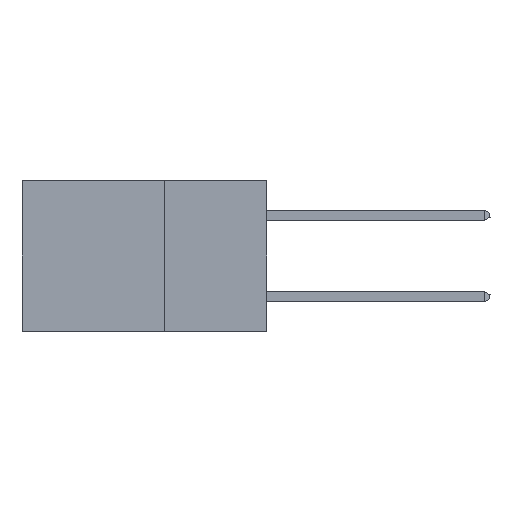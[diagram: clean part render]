
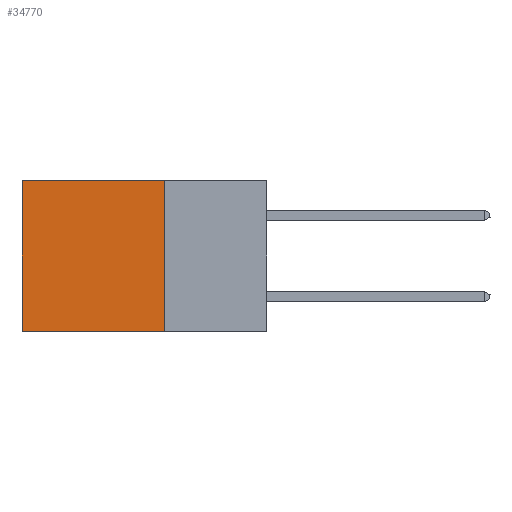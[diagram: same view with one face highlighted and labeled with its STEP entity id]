
A CAD part, left-side view. The second image highlights one B-rep face of the part: STEP entity #34770.
In plain terms, the highlighted planar face has unit normal (-1, 0, 0).
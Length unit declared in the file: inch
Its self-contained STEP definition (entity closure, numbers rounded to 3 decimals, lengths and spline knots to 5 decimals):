
#224 = LINE ( 'NONE', #38371, #41093 ) ;
#1330 = VECTOR ( 'NONE', #21002, 39.37008 ) ;
#1623 = DIRECTION ( 'NONE',  ( 0., 0., -1. ) ) ;
#4645 = CARTESIAN_POINT ( 'NONE',  ( 0.2875, 0.6, 0. ) ) ;
#5847 = CARTESIAN_POINT ( 'NONE',  ( 0.2875, 0.6, -0.37 ) ) ;
#6607 = LINE ( 'NONE', #7288, #1330 ) ;
#7288 = CARTESIAN_POINT ( 'NONE',  ( 0.2875, 0.6, 0. ) ) ;
#8214 = EDGE_CURVE ( 'NONE', #26000, #24510, #19349, .T. ) ;
#8493 = CARTESIAN_POINT ( 'NONE',  ( 0.2875, 0.25, 0. ) ) ;
#8495 = CARTESIAN_POINT ( 'NONE',  ( 0.2875, 0.25, 0. ) ) ;
#9388 = ORIENTED_EDGE ( 'NONE', *, *, #12309, .T. ) ;
#9783 = VERTEX_POINT ( 'NONE', #44958 ) ;
#10341 = EDGE_CURVE ( 'NONE', #9783, #12881, #25858, .T. ) ;
#10484 = CARTESIAN_POINT ( 'NONE',  ( 0.2875, 0.25, -0.37 ) ) ;
#12309 = EDGE_CURVE ( 'NONE', #12881, #24510, #6607, .T. ) ;
#12881 = VERTEX_POINT ( 'NONE', #4645 ) ;
#15265 = AXIS2_PLACEMENT_3D ( 'NONE', #8495, #32923, #1623 ) ;
#16148 = CARTESIAN_POINT ( 'NONE',  ( 0.2875, 0.25, -0.37 ) ) ;
#16545 = ORIENTED_EDGE ( 'NONE', *, *, #19852, .F. ) ;
#18821 = ORIENTED_EDGE ( 'NONE', *, *, #8214, .F. ) ;
#19349 = LINE ( 'NONE', #16148, #43800 ) ;
#19852 = EDGE_CURVE ( 'NONE', #9783, #26000, #224, .T. ) ;
#21002 = DIRECTION ( 'NONE',  ( 0., 0., -1. ) ) ;
#22776 = DIRECTION ( 'NONE',  ( 0., 1., 0. ) ) ;
#24510 = VERTEX_POINT ( 'NONE', #5847 ) ;
#25858 = LINE ( 'NONE', #8493, #29210 ) ;
#26000 = VERTEX_POINT ( 'NONE', #10484 ) ;
#29210 = VECTOR ( 'NONE', #40023, 39.37008 ) ;
#32523 = ORIENTED_EDGE ( 'NONE', *, *, #10341, .T. ) ;
#32923 = DIRECTION ( 'NONE',  ( 1., 0., 0. ) ) ;
#34770 = ADVANCED_FACE ( 'NONE', ( #36373 ), #40251, .F. ) ;
#36373 = FACE_OUTER_BOUND ( 'NONE', #39045, .T. ) ;
#38371 = CARTESIAN_POINT ( 'NONE',  ( 0.2875, 0.25, 0. ) ) ;
#39045 = EDGE_LOOP ( 'NONE', ( #9388, #18821, #16545, #32523 ) ) ;
#39046 = DIRECTION ( 'NONE',  ( 0., 0., -1. ) ) ;
#40023 = DIRECTION ( 'NONE',  ( 0., 1., 0. ) ) ;
#40251 = PLANE ( 'NONE',  #15265 ) ;
#41093 = VECTOR ( 'NONE', #39046, 39.37008 ) ;
#43800 = VECTOR ( 'NONE', #22776, 39.37008 ) ;
#44958 = CARTESIAN_POINT ( 'NONE',  ( 0.2875, 0.25, 0. ) ) ;
